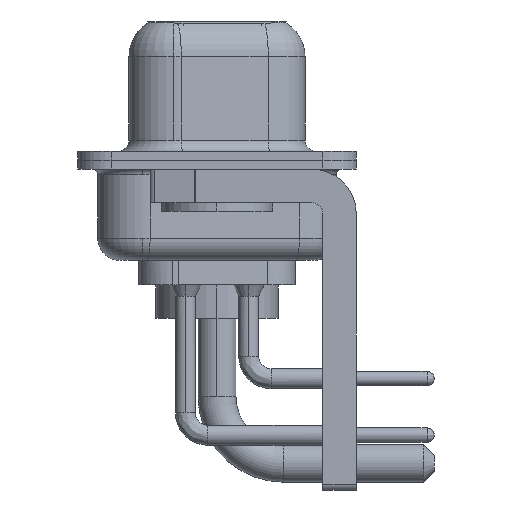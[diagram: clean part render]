
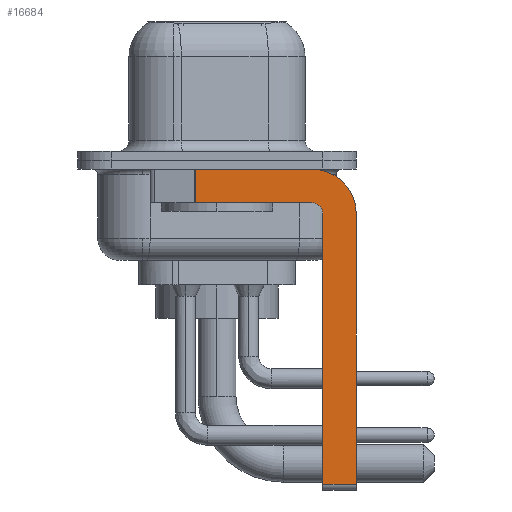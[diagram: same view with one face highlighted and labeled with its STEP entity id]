
A CAD part, left-side view. The second image highlights one B-rep face of the part: STEP entity #16684.
In plain terms, the highlighted planar face has unit normal (-1, 0, 0).
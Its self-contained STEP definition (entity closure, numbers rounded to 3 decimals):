
#951 = EDGE_CURVE ( 'NONE', #6002, #10036, #2603, .T. ) ;
#1179 = CARTESIAN_POINT ( 'NONE',  ( -2.9, 3., -0.4 ) ) ;
#1455 = CARTESIAN_POINT ( 'NONE',  ( -2.9, -6.25, -2.4 ) ) ;
#1820 = VECTOR ( 'NONE', #6439, 1000. ) ;
#2278 = EDGE_CURVE ( 'NONE', #10036, #12950, #15987, .T. ) ;
#2463 = CARTESIAN_POINT ( 'NONE',  ( -2.9, -4.75, -2.4 ) ) ;
#2519 = ORIENTED_EDGE ( 'NONE', *, *, #6125, .F. ) ;
#2585 = CARTESIAN_POINT ( 'NONE',  ( -2.9, -4.25, -1.9 ) ) ;
#2603 = CIRCLE ( 'NONE', #5353, 0.5 ) ;
#3273 = VERTEX_POINT ( 'NONE', #8298 ) ;
#3334 = VECTOR ( 'NONE', #11216, 1000. ) ;
#3425 = EDGE_LOOP ( 'NONE', ( #16171, #16304, #7737, #15122, #12112, #6603, #6764, #2519 ) ) ;
#3506 = CARTESIAN_POINT ( 'NONE',  ( -2.9, -4.25, -14.55 ) ) ;
#3542 = LINE ( 'NONE', #10365, #4897 ) ;
#4897 = VECTOR ( 'NONE', #10110, 1000. ) ;
#5262 = DIRECTION ( 'NONE',  ( 0., 1., 0. ) ) ;
#5353 = AXIS2_PLACEMENT_3D ( 'NONE', #11968, #9114, #9370 ) ;
#5720 = VECTOR ( 'NONE', #5262, 1000. ) ;
#5931 = CARTESIAN_POINT ( 'NONE',  ( -2.9, -4.25, -2.4 ) ) ;
#6002 = VERTEX_POINT ( 'NONE', #2463 ) ;
#6120 = CARTESIAN_POINT ( 'NONE',  ( -2.9, -6.25, -14.55 ) ) ;
#6125 = EDGE_CURVE ( 'NONE', #3273, #13800, #11617, .T. ) ;
#6354 = LINE ( 'NONE', #1179, #1820 ) ;
#6439 = DIRECTION ( 'NONE',  ( 0., -1., 0. ) ) ;
#6603 = ORIENTED_EDGE ( 'NONE', *, *, #10042, .T. ) ;
#6721 = EDGE_CURVE ( 'NONE', #13800, #16284, #8534, .T. ) ;
#6764 = ORIENTED_EDGE ( 'NONE', *, *, #6721, .F. ) ;
#7129 = VERTEX_POINT ( 'NONE', #11813 ) ;
#7200 = LINE ( 'NONE', #15057, #10261 ) ;
#7323 = CARTESIAN_POINT ( 'NONE',  ( -2.9, -6.25, -2.4 ) ) ;
#7602 = EDGE_CURVE ( 'NONE', #7129, #12950, #7200, .T. ) ;
#7737 = ORIENTED_EDGE ( 'NONE', *, *, #2278, .F. ) ;
#7877 = CARTESIAN_POINT ( 'NONE',  ( -2.9, 0.978, -1.9 ) ) ;
#8298 = CARTESIAN_POINT ( 'NONE',  ( -2.9, -4.25, -0.4 ) ) ;
#8305 = CARTESIAN_POINT ( 'NONE',  ( -2.9, -4.25, -2.4 ) ) ;
#8388 = DIRECTION ( 'NONE',  ( 0., 0., -1. ) ) ;
#8399 = DIRECTION ( 'NONE',  ( 0., 0., -1. ) ) ;
#8534 = LINE ( 'NONE', #7323, #3334 ) ;
#9114 = DIRECTION ( 'NONE',  ( -1., 0., 0. ) ) ;
#9370 = DIRECTION ( 'NONE',  ( 0., 0., 1. ) ) ;
#9668 = DIRECTION ( 'NONE',  ( 1., 0., 0. ) ) ;
#10036 = VERTEX_POINT ( 'NONE', #15589 ) ;
#10042 = EDGE_CURVE ( 'NONE', #10100, #16284, #14303, .T. ) ;
#10100 = VERTEX_POINT ( 'NONE', #16102 ) ;
#10110 = DIRECTION ( 'NONE',  ( 0., 0., 1. ) ) ;
#10261 = VECTOR ( 'NONE', #8399, 1000. ) ;
#10365 = CARTESIAN_POINT ( 'NONE',  ( -2.9, -4.75, -14.8 ) ) ;
#11039 = FACE_OUTER_BOUND ( 'NONE', #3425, .T. ) ;
#11209 = DIRECTION ( 'NONE',  ( 0., 0., -1. ) ) ;
#11216 = DIRECTION ( 'NONE',  ( 0., 0., -1. ) ) ;
#11345 = VECTOR ( 'NONE', #14055, 1000. ) ;
#11617 = CIRCLE ( 'NONE', #13839, 2. ) ;
#11813 = CARTESIAN_POINT ( 'NONE',  ( -2.9, 0.978, -0.4 ) ) ;
#11968 = CARTESIAN_POINT ( 'NONE',  ( -2.9, -4.25, -2.4 ) ) ;
#12112 = ORIENTED_EDGE ( 'NONE', *, *, #16415, .F. ) ;
#12302 = DIRECTION ( 'NONE',  ( 1., 0., 0. ) ) ;
#12950 = VERTEX_POINT ( 'NONE', #7877 ) ;
#13800 = VERTEX_POINT ( 'NONE', #1455 ) ;
#13839 = AXIS2_PLACEMENT_3D ( 'NONE', #8305, #12302, #8388 ) ;
#14055 = DIRECTION ( 'NONE',  ( 0., -1., 0. ) ) ;
#14303 = LINE ( 'NONE', #3506, #11345 ) ;
#14352 = EDGE_CURVE ( 'NONE', #7129, #3273, #6354, .T. ) ;
#15057 = CARTESIAN_POINT ( 'NONE',  ( -2.9, 0.978, -1.9 ) ) ;
#15122 = ORIENTED_EDGE ( 'NONE', *, *, #951, .F. ) ;
#15589 = CARTESIAN_POINT ( 'NONE',  ( -2.9, -4.25, -1.9 ) ) ;
#15987 = LINE ( 'NONE', #2585, #5720 ) ;
#16102 = CARTESIAN_POINT ( 'NONE',  ( -2.9, -4.75, -14.55 ) ) ;
#16171 = ORIENTED_EDGE ( 'NONE', *, *, #14352, .F. ) ;
#16219 = PLANE ( 'NONE',  #17060 ) ;
#16284 = VERTEX_POINT ( 'NONE', #6120 ) ;
#16304 = ORIENTED_EDGE ( 'NONE', *, *, #7602, .T. ) ;
#16415 = EDGE_CURVE ( 'NONE', #10100, #6002, #3542, .T. ) ;
#16684 = ADVANCED_FACE ( 'NONE', ( #11039 ), #16219, .F. ) ;
#17060 = AXIS2_PLACEMENT_3D ( 'NONE', #5931, #9668, #11209 ) ;
